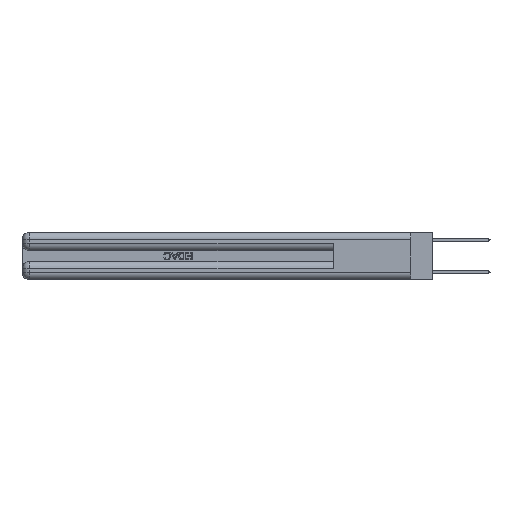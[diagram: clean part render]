
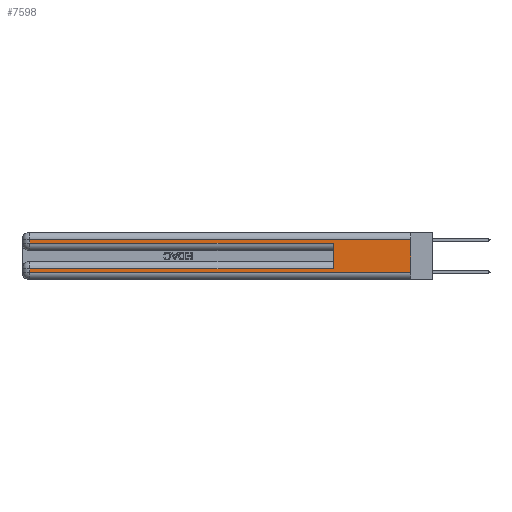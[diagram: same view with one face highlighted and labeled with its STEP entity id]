
A CAD part, left-side view. The second image highlights one B-rep face of the part: STEP entity #7598.
In plain terms, the highlighted planar face has unit normal (-1, 0, 0).
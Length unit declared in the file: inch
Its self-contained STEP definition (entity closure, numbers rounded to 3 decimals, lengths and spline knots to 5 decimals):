
#153 = LINE ( 'NONE', #692, #11773 ) ;
#446 = CARTESIAN_POINT ( 'NONE',  ( 0., 2.94, 0.37 ) ) ;
#676 = EDGE_CURVE ( 'NONE', #9657, #23200, #153, .T. ) ;
#692 = CARTESIAN_POINT ( 'NONE',  ( 0., 0., 0.37 ) ) ;
#1541 = VECTOR ( 'NONE', #3212, 39.37008 ) ;
#1938 = AXIS2_PLACEMENT_3D ( 'NONE', #5097, #20968, #32148 ) ;
#3212 = DIRECTION ( 'NONE',  ( 0., -1., 0. ) ) ;
#3852 = VECTOR ( 'NONE', #21092, 39.37008 ) ;
#4895 = VERTEX_POINT ( 'NONE', #19477 ) ;
#5097 = CARTESIAN_POINT ( 'NONE',  ( 0., 0., 0.37 ) ) ;
#5857 = EDGE_CURVE ( 'NONE', #4895, #21944, #23003, .T. ) ;
#6092 = LINE ( 'NONE', #9561, #23843 ) ;
#6739 = LINE ( 'NONE', #12263, #15834 ) ;
#7598 = ADVANCED_FACE ( 'NONE', ( #19069 ), #30265, .F. ) ;
#8720 = CARTESIAN_POINT ( 'NONE',  ( 0., 0., 0.285 ) ) ;
#9561 = CARTESIAN_POINT ( 'NONE',  ( 0., 0., 0.06 ) ) ;
#9657 = VERTEX_POINT ( 'NONE', #19629 ) ;
#11229 = EDGE_CURVE ( 'NONE', #4895, #30032, #34841, .T. ) ;
#11564 = EDGE_CURVE ( 'NONE', #21944, #12473, #33715, .T. ) ;
#11773 = VECTOR ( 'NONE', #33968, 39.37008 ) ;
#12113 = VERTEX_POINT ( 'NONE', #24316 ) ;
#12147 = DIRECTION ( 'NONE',  ( 0., -1., 0. ) ) ;
#12263 = CARTESIAN_POINT ( 'NONE',  ( 0., 2.94, 0.37 ) ) ;
#12473 = VERTEX_POINT ( 'NONE', #33831 ) ;
#12491 = ORIENTED_EDGE ( 'NONE', *, *, #676, .F. ) ;
#14635 = ORIENTED_EDGE ( 'NONE', *, *, #31523, .T. ) ;
#14659 = EDGE_LOOP ( 'NONE', ( #12491, #33809, #19815, #14635, #28898, #32257, #14769, #35512 ) ) ;
#14769 = ORIENTED_EDGE ( 'NONE', *, *, #11564, .T. ) ;
#15752 = CARTESIAN_POINT ( 'NONE',  ( 0., 0.6, 0.145 ) ) ;
#15834 = VECTOR ( 'NONE', #17969, 39.37008 ) ;
#15920 = CARTESIAN_POINT ( 'NONE',  ( 0., 0.6, 0.285 ) ) ;
#17969 = DIRECTION ( 'NONE',  ( 0., 0., -1. ) ) ;
#18959 = CARTESIAN_POINT ( 'NONE',  ( 0., 2.94, 0.31 ) ) ;
#19069 = FACE_OUTER_BOUND ( 'NONE', #14659, .T. ) ;
#19477 = CARTESIAN_POINT ( 'NONE',  ( 0., 0.6, 0.085 ) ) ;
#19629 = CARTESIAN_POINT ( 'NONE',  ( 0., 0., 0.31 ) ) ;
#19815 = ORIENTED_EDGE ( 'NONE', *, *, #22619, .T. ) ;
#20968 = DIRECTION ( 'NONE',  ( 1., 0., 0. ) ) ;
#20981 = DIRECTION ( 'NONE',  ( 0., 1., 0. ) ) ;
#21092 = DIRECTION ( 'NONE',  ( 0., 0., 1. ) ) ;
#21944 = VERTEX_POINT ( 'NONE', #34576 ) ;
#22619 = EDGE_CURVE ( 'NONE', #29260, #12113, #6739, .T. ) ;
#22907 = LINE ( 'NONE', #23453, #26248 ) ;
#23003 = LINE ( 'NONE', #23552, #24243 ) ;
#23200 = VERTEX_POINT ( 'NONE', #32928 ) ;
#23453 = CARTESIAN_POINT ( 'NONE',  ( 0., 0., 0.31 ) ) ;
#23552 = CARTESIAN_POINT ( 'NONE',  ( 0., 0., 0.085 ) ) ;
#23843 = VECTOR ( 'NONE', #12147, 39.37008 ) ;
#24243 = VECTOR ( 'NONE', #20981, 39.37008 ) ;
#24316 = CARTESIAN_POINT ( 'NONE',  ( 0., 2.94, 0.285 ) ) ;
#26248 = VECTOR ( 'NONE', #34256, 39.37008 ) ;
#28898 = ORIENTED_EDGE ( 'NONE', *, *, #11229, .F. ) ;
#29151 = EDGE_CURVE ( 'NONE', #12473, #23200, #6092, .T. ) ;
#29260 = VERTEX_POINT ( 'NONE', #18959 ) ;
#30032 = VERTEX_POINT ( 'NONE', #15920 ) ;
#30265 = PLANE ( 'NONE',  #1938 ) ;
#31490 = LINE ( 'NONE', #8720, #1541 ) ;
#31523 = EDGE_CURVE ( 'NONE', #12113, #30032, #31490, .T. ) ;
#32148 = DIRECTION ( 'NONE',  ( 0., 0., -1. ) ) ;
#32257 = ORIENTED_EDGE ( 'NONE', *, *, #5857, .T. ) ;
#32928 = CARTESIAN_POINT ( 'NONE',  ( 0., 0., 0.06 ) ) ;
#33156 = EDGE_CURVE ( 'NONE', #9657, #29260, #22907, .T. ) ;
#33715 = LINE ( 'NONE', #446, #34272 ) ;
#33809 = ORIENTED_EDGE ( 'NONE', *, *, #33156, .T. ) ;
#33831 = CARTESIAN_POINT ( 'NONE',  ( 0., 2.94, 0.06 ) ) ;
#33968 = DIRECTION ( 'NONE',  ( 0., 0., -1. ) ) ;
#34071 = DIRECTION ( 'NONE',  ( 0., 0., -1. ) ) ;
#34256 = DIRECTION ( 'NONE',  ( 0., 1., 0. ) ) ;
#34272 = VECTOR ( 'NONE', #34071, 39.37008 ) ;
#34576 = CARTESIAN_POINT ( 'NONE',  ( 0., 2.94, 0.085 ) ) ;
#34841 = LINE ( 'NONE', #15752, #3852 ) ;
#35512 = ORIENTED_EDGE ( 'NONE', *, *, #29151, .T. ) ;
